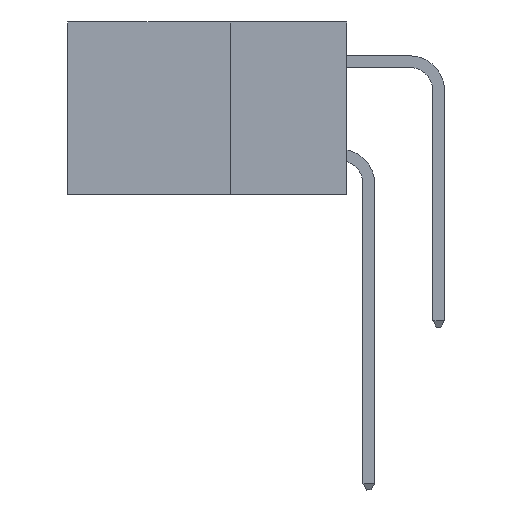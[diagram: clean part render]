
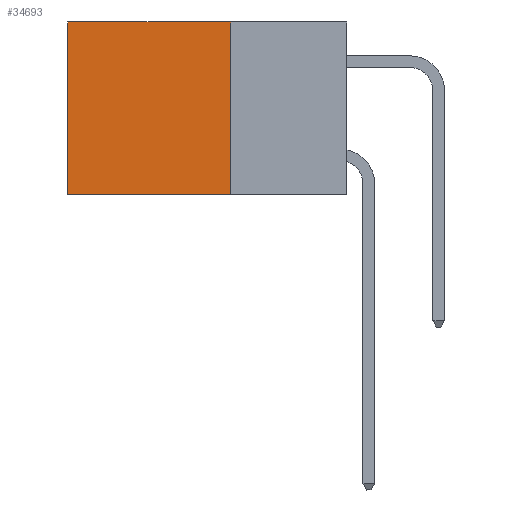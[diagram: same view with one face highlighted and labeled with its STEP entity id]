
A CAD part, left-side view. The second image highlights one B-rep face of the part: STEP entity #34693.
In plain terms, the highlighted planar face has unit normal (-1, 0, 0).
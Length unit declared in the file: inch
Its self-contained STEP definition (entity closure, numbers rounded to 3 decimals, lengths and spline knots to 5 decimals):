
#2195 = CARTESIAN_POINT ( 'NONE',  ( 0.2875, 0.6, -0.37 ) ) ;
#2233 = EDGE_CURVE ( 'NONE', #14657, #4972, #43195, .T. ) ;
#3145 = DIRECTION ( 'NONE',  ( 0., 1., 0. ) ) ;
#3452 = DIRECTION ( 'NONE',  ( 0., 1., 0. ) ) ;
#4326 = CARTESIAN_POINT ( 'NONE',  ( 0.2875, 0.25, -0.37 ) ) ;
#4629 = EDGE_CURVE ( 'NONE', #4972, #10003, #27269, .T. ) ;
#4972 = VERTEX_POINT ( 'NONE', #26343 ) ;
#5994 = FACE_OUTER_BOUND ( 'NONE', #28025, .T. ) ;
#6849 = AXIS2_PLACEMENT_3D ( 'NONE', #33281, #19848, #9585 ) ;
#7160 = DIRECTION ( 'NONE',  ( 0., 0., -1. ) ) ;
#9585 = DIRECTION ( 'NONE',  ( 0., 0., -1. ) ) ;
#9839 = CARTESIAN_POINT ( 'NONE',  ( 0.2875, 0.6, 0. ) ) ;
#10003 = VERTEX_POINT ( 'NONE', #2195 ) ;
#11039 = LINE ( 'NONE', #4326, #37989 ) ;
#13305 = ORIENTED_EDGE ( 'NONE', *, *, #43829, .F. ) ;
#14657 = VERTEX_POINT ( 'NONE', #28624 ) ;
#18321 = VECTOR ( 'NONE', #3145, 39.37008 ) ;
#19208 = LINE ( 'NONE', #30163, #43546 ) ;
#19848 = DIRECTION ( 'NONE',  ( 1., 0., 0. ) ) ;
#26343 = CARTESIAN_POINT ( 'NONE',  ( 0.2875, 0.6, 0. ) ) ;
#27269 = LINE ( 'NONE', #9839, #38074 ) ;
#28025 = EDGE_LOOP ( 'NONE', ( #42952, #13305, #33247, #43006 ) ) ;
#28624 = CARTESIAN_POINT ( 'NONE',  ( 0.2875, 0.25, 0. ) ) ;
#30163 = CARTESIAN_POINT ( 'NONE',  ( 0.2875, 0.25, 0. ) ) ;
#31421 = EDGE_CURVE ( 'NONE', #14657, #43931, #19208, .T. ) ;
#33247 = ORIENTED_EDGE ( 'NONE', *, *, #31421, .F. ) ;
#33281 = CARTESIAN_POINT ( 'NONE',  ( 0.2875, 0.25, 0. ) ) ;
#34693 = ADVANCED_FACE ( 'NONE', ( #5994 ), #36840, .F. ) ;
#35388 = CARTESIAN_POINT ( 'NONE',  ( 0.2875, 0.25, -0.37 ) ) ;
#36840 = PLANE ( 'NONE',  #6849 ) ;
#37989 = VECTOR ( 'NONE', #3452, 39.37008 ) ;
#38074 = VECTOR ( 'NONE', #7160, 39.37008 ) ;
#39598 = CARTESIAN_POINT ( 'NONE',  ( 0.2875, 0.25, 0. ) ) ;
#39996 = DIRECTION ( 'NONE',  ( 0., 0., -1. ) ) ;
#42952 = ORIENTED_EDGE ( 'NONE', *, *, #4629, .T. ) ;
#43006 = ORIENTED_EDGE ( 'NONE', *, *, #2233, .T. ) ;
#43195 = LINE ( 'NONE', #39598, #18321 ) ;
#43546 = VECTOR ( 'NONE', #39996, 39.37008 ) ;
#43829 = EDGE_CURVE ( 'NONE', #43931, #10003, #11039, .T. ) ;
#43931 = VERTEX_POINT ( 'NONE', #35388 ) ;
